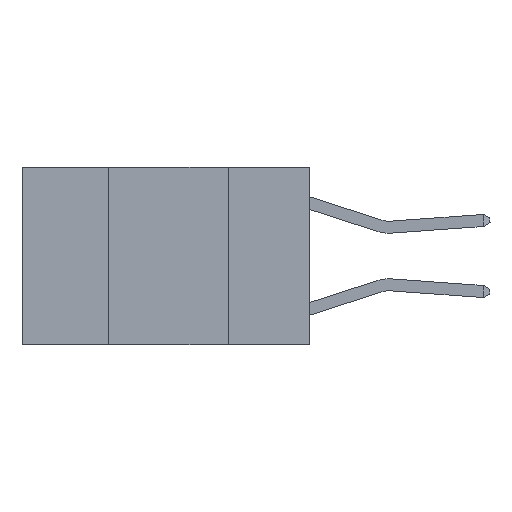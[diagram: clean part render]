
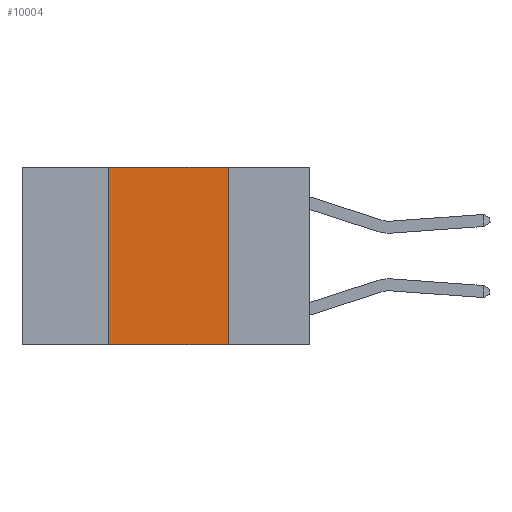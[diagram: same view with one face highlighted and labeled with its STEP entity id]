
A CAD part, left-side view. The second image highlights one B-rep face of the part: STEP entity #10004.
In plain terms, the highlighted planar face has unit normal (-1, 0, 0).
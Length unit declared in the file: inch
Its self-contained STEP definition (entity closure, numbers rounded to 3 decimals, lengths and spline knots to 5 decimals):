
#345 = LINE ( 'NONE', #13082, #11079 ) ;
#1338 = VERTEX_POINT ( 'NONE', #1711 ) ;
#1711 = CARTESIAN_POINT ( 'NONE',  ( 0., 0.42, -0.37 ) ) ;
#2066 = DIRECTION ( 'NONE',  ( 0., -1., 0. ) ) ;
#2820 = CARTESIAN_POINT ( 'NONE',  ( 0., 0.42, 0. ) ) ;
#3191 = VERTEX_POINT ( 'NONE', #2820 ) ;
#3332 = CARTESIAN_POINT ( 'NONE',  ( 0., 0.42, 0. ) ) ;
#3392 = EDGE_LOOP ( 'NONE', ( #13541, #9647, #12190, #5203 ) ) ;
#4147 = PLANE ( 'NONE',  #12391 ) ;
#4457 = VERTEX_POINT ( 'NONE', #5650 ) ;
#5203 = ORIENTED_EDGE ( 'NONE', *, *, #8769, .T. ) ;
#5650 = CARTESIAN_POINT ( 'NONE',  ( 0., 0.17, -0.37 ) ) ;
#6221 = LINE ( 'NONE', #10438, #11426 ) ;
#6375 = DIRECTION ( 'NONE',  ( 0., 0., -1. ) ) ;
#6514 = CARTESIAN_POINT ( 'NONE',  ( 0., 0.17, 0. ) ) ;
#7854 = VERTEX_POINT ( 'NONE', #6514 ) ;
#8344 = EDGE_CURVE ( 'NONE', #7854, #4457, #6221, .T. ) ;
#8568 = EDGE_CURVE ( 'NONE', #1338, #3191, #11886, .T. ) ;
#8571 = VECTOR ( 'NONE', #8789, 39.37008 ) ;
#8769 = EDGE_CURVE ( 'NONE', #1338, #4457, #345, .T. ) ;
#8789 = DIRECTION ( 'NONE',  ( 0., 0., 1. ) ) ;
#9328 = FACE_OUTER_BOUND ( 'NONE', #3392, .T. ) ;
#9647 = ORIENTED_EDGE ( 'NONE', *, *, #10081, .F. ) ;
#10004 = ADVANCED_FACE ( 'NONE', ( #9328 ), #4147, .F. ) ;
#10081 = EDGE_CURVE ( 'NONE', #3191, #7854, #11059, .T. ) ;
#10115 = DIRECTION ( 'NONE',  ( 0., -1., 0. ) ) ;
#10438 = CARTESIAN_POINT ( 'NONE',  ( 0., 0.17, 0. ) ) ;
#10629 = CARTESIAN_POINT ( 'NONE',  ( 0., 0.6, 0. ) ) ;
#11059 = LINE ( 'NONE', #10629, #13365 ) ;
#11079 = VECTOR ( 'NONE', #10115, 39.37008 ) ;
#11426 = VECTOR ( 'NONE', #11479, 39.37008 ) ;
#11479 = DIRECTION ( 'NONE',  ( 0., 0., -1. ) ) ;
#11534 = CARTESIAN_POINT ( 'NONE',  ( 0., 0.6, 0. ) ) ;
#11886 = LINE ( 'NONE', #3332, #8571 ) ;
#12190 = ORIENTED_EDGE ( 'NONE', *, *, #8568, .F. ) ;
#12391 = AXIS2_PLACEMENT_3D ( 'NONE', #11534, #12513, #6375 ) ;
#12513 = DIRECTION ( 'NONE',  ( 1., 0., 0. ) ) ;
#13082 = CARTESIAN_POINT ( 'NONE',  ( 0., 0.6, -0.37 ) ) ;
#13365 = VECTOR ( 'NONE', #2066, 39.37008 ) ;
#13541 = ORIENTED_EDGE ( 'NONE', *, *, #8344, .F. ) ;
